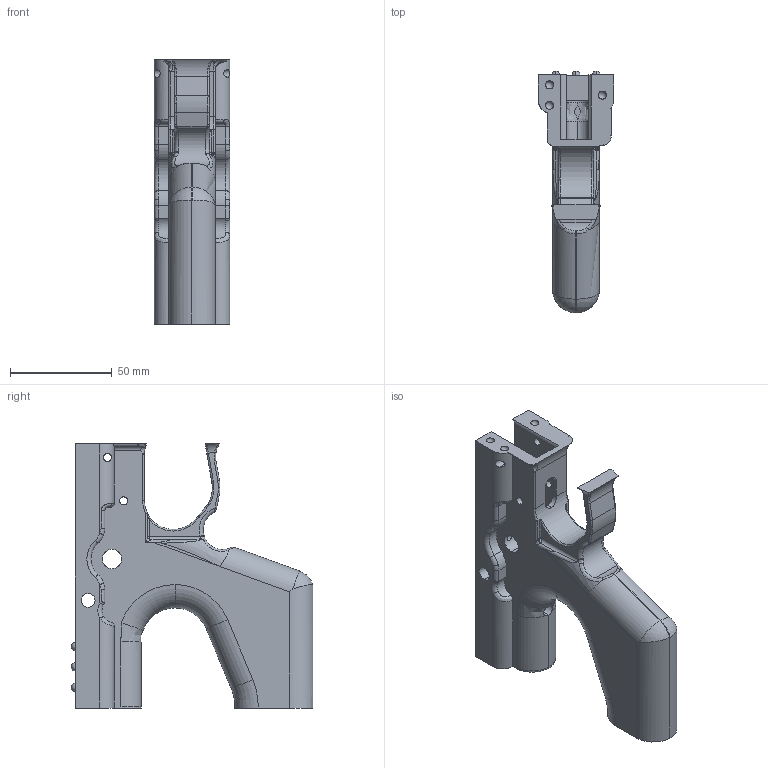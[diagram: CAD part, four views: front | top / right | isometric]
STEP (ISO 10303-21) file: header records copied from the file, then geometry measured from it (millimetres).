
FILE_DESCRIPTION (( 'STEP AP214' ), '1' );
FILE_NAME ('Grip_2.STEP', '2015-10-23T19:39:34', ( 'WarFairy' ), ( '' ), 'SwSTEP 2.0', 'SolidWorks 2015', '' );
FILE_SCHEMA (( 'AUTOMOTIVE_DESIGN' ));
Length unit declared in the file: millimetre
Products named in the file (1): Grip_2
Bounding box: 37.13 x 119.02 x 130 mm (x, y, z)
Volume: 190710.3 mm3; surface area: 40634.6 mm2
Topology: 1 solids, 1 shells, 299 faces, 850 edges, 520 vertices
Faces by surface type: cylinder 109, bspline 59, sphere 47, torus 44, plane 40
Entity records: 13484 total; most frequent: CARTESIAN_POINT 6614, ORIENTED_EDGE 1502, DIRECTION 1357, EDGE_CURVE 751, AXIS2_PLACEMENT_3D 571, VERTEX_POINT 474, EDGE_LOOP 341, CIRCLE 330
